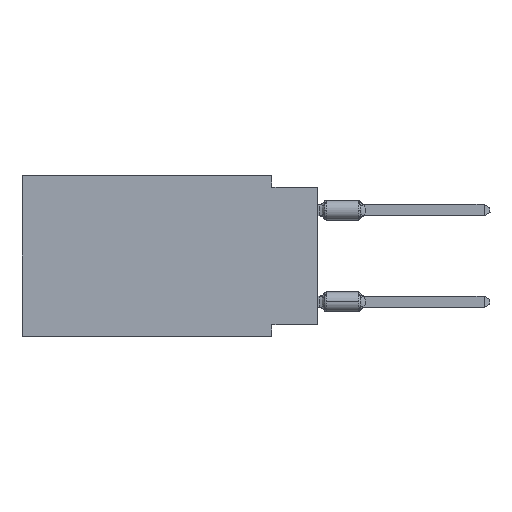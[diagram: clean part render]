
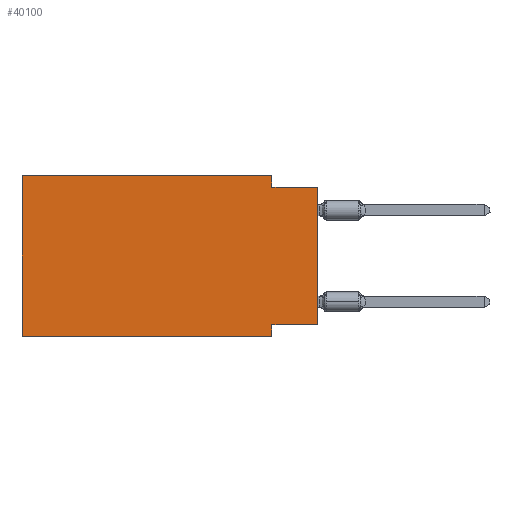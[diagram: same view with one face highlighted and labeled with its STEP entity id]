
A CAD part, left-side view. The second image highlights one B-rep face of the part: STEP entity #40100.
In plain terms, the highlighted planar face has unit normal (-1, 0, 0).
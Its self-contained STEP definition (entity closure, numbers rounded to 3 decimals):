
#1137 = DIRECTION ( 'NONE',  ( 0., 0., 1. ) ) ;
#2213 = CARTESIAN_POINT ( 'NONE',  ( 0., 16.383, 0. ) ) ;
#4151 = AXIS2_PLACEMENT_3D ( 'NONE', #19071, #24322, #61011 ) ;
#4248 = ORIENTED_EDGE ( 'NONE', *, *, #42001, .F. ) ;
#6005 = CARTESIAN_POINT ( 'NONE',  ( 0., 0., -0.635 ) ) ;
#8609 = VERTEX_POINT ( 'NONE', #6005 ) ;
#10628 = CARTESIAN_POINT ( 'NONE',  ( 0., 2.54, 0. ) ) ;
#10819 = CARTESIAN_POINT ( 'NONE',  ( 0., 0., -0.635 ) ) ;
#10928 = LINE ( 'NONE', #10628, #40633 ) ;
#11662 = DIRECTION ( 'NONE',  ( 0., 0., -1. ) ) ;
#13168 = LINE ( 'NONE', #35851, #28195 ) ;
#13750 = ORIENTED_EDGE ( 'NONE', *, *, #38139, .T. ) ;
#14389 = VERTEX_POINT ( 'NONE', #47460 ) ;
#14881 = DIRECTION ( 'NONE',  ( 0., -1., 0. ) ) ;
#17135 = VERTEX_POINT ( 'NONE', #18720 ) ;
#18720 = CARTESIAN_POINT ( 'NONE',  ( 0., 16.383, 0. ) ) ;
#18771 = FACE_OUTER_BOUND ( 'NONE', #33026, .T. ) ;
#19071 = CARTESIAN_POINT ( 'NONE',  ( 0., 16.383, 0. ) ) ;
#19283 = VECTOR ( 'NONE', #24670, 1000. ) ;
#20256 = LINE ( 'NONE', #2213, #29235 ) ;
#20551 = EDGE_CURVE ( 'NONE', #50753, #36411, #50451, .T. ) ;
#22212 = CARTESIAN_POINT ( 'NONE',  ( 0., 2.54, -8.89 ) ) ;
#22318 = LINE ( 'NONE', #60836, #24636 ) ;
#24322 = DIRECTION ( 'NONE',  ( 1., 0., 0. ) ) ;
#24378 = VERTEX_POINT ( 'NONE', #39212 ) ;
#24636 = VECTOR ( 'NONE', #41584, 1000. ) ;
#24670 = DIRECTION ( 'NONE',  ( 0., 1., 0. ) ) ;
#24805 = ORIENTED_EDGE ( 'NONE', *, *, #55552, .F. ) ;
#25407 = EDGE_CURVE ( 'NONE', #59688, #36411, #13168, .T. ) ;
#26396 = EDGE_CURVE ( 'NONE', #17135, #24378, #20256, .T. ) ;
#28067 = ORIENTED_EDGE ( 'NONE', *, *, #26396, .F. ) ;
#28195 = VECTOR ( 'NONE', #36467, 1000. ) ;
#29235 = VECTOR ( 'NONE', #53480, 1000. ) ;
#30221 = EDGE_CURVE ( 'NONE', #14389, #50753, #38964, .T. ) ;
#33026 = EDGE_LOOP ( 'NONE', ( #13750, #24805, #56232, #28067, #4248, #60064, #43031, #60543 ) ) ;
#35851 = CARTESIAN_POINT ( 'NONE',  ( 0., 16.383, -8.89 ) ) ;
#36411 = VERTEX_POINT ( 'NONE', #55955 ) ;
#36467 = DIRECTION ( 'NONE',  ( 0., -1., 0. ) ) ;
#38139 = EDGE_CURVE ( 'NONE', #14389, #8609, #43711, .T. ) ;
#38964 = LINE ( 'NONE', #48251, #19283 ) ;
#39212 = CARTESIAN_POINT ( 'NONE',  ( 0., 2.54, 0. ) ) ;
#40100 = ADVANCED_FACE ( 'NONE', ( #18771 ), #42979, .F. ) ;
#40633 = VECTOR ( 'NONE', #48809, 1000. ) ;
#40642 = VECTOR ( 'NONE', #1137, 1000. ) ;
#41283 = CARTESIAN_POINT ( 'NONE',  ( 0., 16.383, -8.89 ) ) ;
#41584 = DIRECTION ( 'NONE',  ( 0., 0., 1. ) ) ;
#42001 = EDGE_CURVE ( 'NONE', #59688, #17135, #22318, .T. ) ;
#42979 = PLANE ( 'NONE',  #4151 ) ;
#43031 = ORIENTED_EDGE ( 'NONE', *, *, #20551, .F. ) ;
#43571 = CARTESIAN_POINT ( 'NONE',  ( 0., 2.54, -0.635 ) ) ;
#43711 = LINE ( 'NONE', #44315, #40642 ) ;
#44315 = CARTESIAN_POINT ( 'NONE',  ( 0., 0., 0. ) ) ;
#46681 = VECTOR ( 'NONE', #11662, 1000. ) ;
#47460 = CARTESIAN_POINT ( 'NONE',  ( 0., 0., -8.255 ) ) ;
#47548 = VECTOR ( 'NONE', #14881, 1000. ) ;
#48059 = EDGE_CURVE ( 'NONE', #24378, #56878, #10928, .T. ) ;
#48251 = CARTESIAN_POINT ( 'NONE',  ( 0., 0., -8.255 ) ) ;
#48809 = DIRECTION ( 'NONE',  ( 0., 0., -1. ) ) ;
#50451 = LINE ( 'NONE', #22212, #46681 ) ;
#50753 = VERTEX_POINT ( 'NONE', #56942 ) ;
#53362 = LINE ( 'NONE', #10819, #47548 ) ;
#53480 = DIRECTION ( 'NONE',  ( 0., -1., 0. ) ) ;
#55552 = EDGE_CURVE ( 'NONE', #56878, #8609, #53362, .T. ) ;
#55955 = CARTESIAN_POINT ( 'NONE',  ( 0., 2.54, -8.89 ) ) ;
#56232 = ORIENTED_EDGE ( 'NONE', *, *, #48059, .F. ) ;
#56878 = VERTEX_POINT ( 'NONE', #43571 ) ;
#56942 = CARTESIAN_POINT ( 'NONE',  ( 0., 2.54, -8.255 ) ) ;
#59688 = VERTEX_POINT ( 'NONE', #41283 ) ;
#60064 = ORIENTED_EDGE ( 'NONE', *, *, #25407, .T. ) ;
#60543 = ORIENTED_EDGE ( 'NONE', *, *, #30221, .F. ) ;
#60836 = CARTESIAN_POINT ( 'NONE',  ( 0., 16.383, 0. ) ) ;
#61011 = DIRECTION ( 'NONE',  ( 0., 0., -1. ) ) ;
